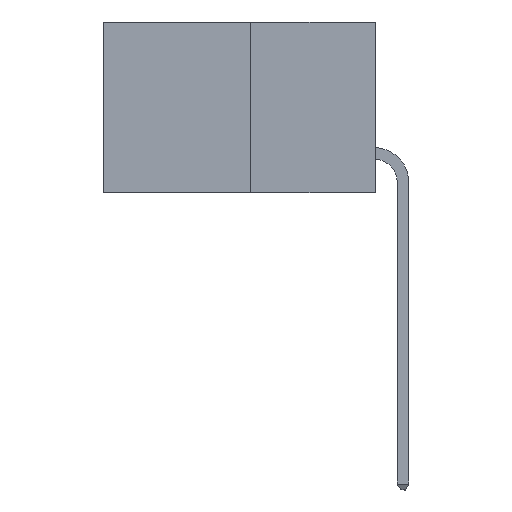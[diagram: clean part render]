
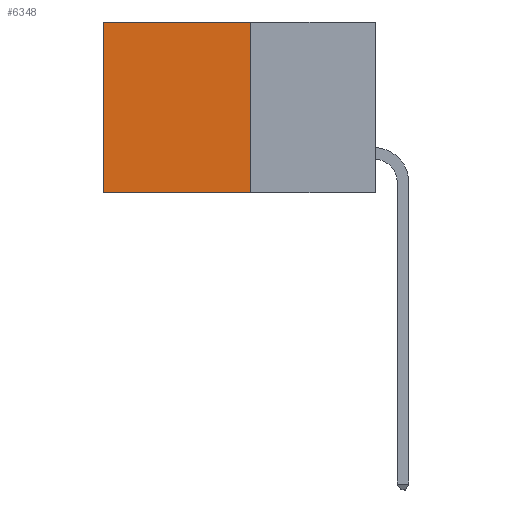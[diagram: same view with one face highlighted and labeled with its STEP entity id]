
A CAD part, left-side view. The second image highlights one B-rep face of the part: STEP entity #6348.
In plain terms, the highlighted planar face has unit normal (-1, 0, 0).
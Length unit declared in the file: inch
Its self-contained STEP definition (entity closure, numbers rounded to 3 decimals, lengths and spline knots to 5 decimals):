
#49 = CARTESIAN_POINT ( 'NONE',  ( 0.277, 0.59, -0.37 ) ) ;
#342 = VERTEX_POINT ( 'NONE', #655 ) ;
#655 = CARTESIAN_POINT ( 'NONE',  ( 0.277, 0.27, 0. ) ) ;
#863 = VECTOR ( 'NONE', #4311, 39.37008 ) ;
#1417 = EDGE_CURVE ( 'NONE', #12384, #5184, #9983, .T. ) ;
#1452 = ORIENTED_EDGE ( 'NONE', *, *, #12462, .T. ) ;
#1795 = AXIS2_PLACEMENT_3D ( 'NONE', #7900, #5894, #14441 ) ;
#2008 = ORIENTED_EDGE ( 'NONE', *, *, #1417, .F. ) ;
#2110 = CARTESIAN_POINT ( 'NONE',  ( 0.277, 0.27, -0.37 ) ) ;
#3021 = LINE ( 'NONE', #8705, #6106 ) ;
#3093 = VECTOR ( 'NONE', #6809, 39.37008 ) ;
#4311 = DIRECTION ( 'NONE',  ( 0., 1., 0. ) ) ;
#4670 = EDGE_CURVE ( 'NONE', #342, #8313, #3021, .T. ) ;
#5184 = VERTEX_POINT ( 'NONE', #13756 ) ;
#5894 = DIRECTION ( 'NONE',  ( 1., 0., 0. ) ) ;
#6106 = VECTOR ( 'NONE', #11185, 39.37008 ) ;
#6180 = LINE ( 'NONE', #2110, #3093 ) ;
#6343 = LINE ( 'NONE', #49, #12159 ) ;
#6348 = ADVANCED_FACE ( 'NONE', ( #12907 ), #10791, .F. ) ;
#6809 = DIRECTION ( 'NONE',  ( 0., 0., -1. ) ) ;
#7900 = CARTESIAN_POINT ( 'NONE',  ( 0.277, 0.27, -0.37 ) ) ;
#7987 = CARTESIAN_POINT ( 'NONE',  ( 0.277, 0.27, -0.37 ) ) ;
#8189 = DIRECTION ( 'NONE',  ( 0., 0., -1. ) ) ;
#8313 = VERTEX_POINT ( 'NONE', #11127 ) ;
#8657 = EDGE_LOOP ( 'NONE', ( #1452, #2008, #11908, #11569 ) ) ;
#8705 = CARTESIAN_POINT ( 'NONE',  ( 0.277, 0.27, 0. ) ) ;
#9983 = LINE ( 'NONE', #12363, #863 ) ;
#10791 = PLANE ( 'NONE',  #1795 ) ;
#11127 = CARTESIAN_POINT ( 'NONE',  ( 0.277, 0.59, 0. ) ) ;
#11185 = DIRECTION ( 'NONE',  ( 0., 1., 0. ) ) ;
#11569 = ORIENTED_EDGE ( 'NONE', *, *, #4670, .T. ) ;
#11886 = EDGE_CURVE ( 'NONE', #342, #12384, #6180, .T. ) ;
#11908 = ORIENTED_EDGE ( 'NONE', *, *, #11886, .F. ) ;
#12159 = VECTOR ( 'NONE', #8189, 39.37008 ) ;
#12363 = CARTESIAN_POINT ( 'NONE',  ( 0.277, 0.27, -0.37 ) ) ;
#12384 = VERTEX_POINT ( 'NONE', #7987 ) ;
#12462 = EDGE_CURVE ( 'NONE', #8313, #5184, #6343, .T. ) ;
#12907 = FACE_OUTER_BOUND ( 'NONE', #8657, .T. ) ;
#13756 = CARTESIAN_POINT ( 'NONE',  ( 0.277, 0.59, -0.37 ) ) ;
#14441 = DIRECTION ( 'NONE',  ( 0., 0., -1. ) ) ;
